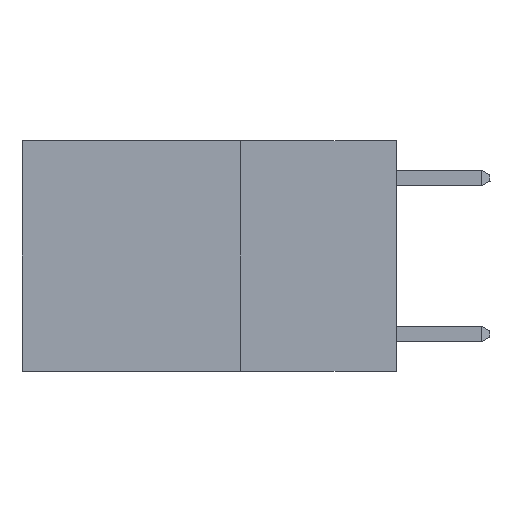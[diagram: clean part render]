
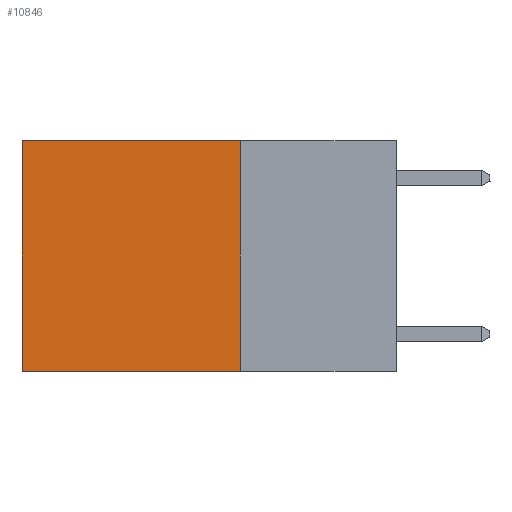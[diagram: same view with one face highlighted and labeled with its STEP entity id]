
A CAD part, left-side view. The second image highlights one B-rep face of the part: STEP entity #10846.
In plain terms, the highlighted planar face has unit normal (-1, 0, 0).
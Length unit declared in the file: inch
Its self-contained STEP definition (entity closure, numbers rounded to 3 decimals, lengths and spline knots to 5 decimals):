
#853 = EDGE_CURVE ( 'NONE', #4057, #1372, #12557, .T. ) ;
#1372 = VERTEX_POINT ( 'NONE', #14731 ) ;
#1392 = FACE_OUTER_BOUND ( 'NONE', #7752, .T. ) ;
#2398 = EDGE_CURVE ( 'NONE', #14390, #4057, #13760, .T. ) ;
#2443 = ORIENTED_EDGE ( 'NONE', *, *, #853, .F. ) ;
#2927 = CARTESIAN_POINT ( 'NONE',  ( 0.2625, 0.25, -0.37 ) ) ;
#2970 = LINE ( 'NONE', #14959, #9417 ) ;
#3280 = ORIENTED_EDGE ( 'NONE', *, *, #3383, .T. ) ;
#3383 = EDGE_CURVE ( 'NONE', #14390, #9085, #14247, .T. ) ;
#3995 = DIRECTION ( 'NONE',  ( 0., 0., -1. ) ) ;
#4057 = VERTEX_POINT ( 'NONE', #10858 ) ;
#6278 = VECTOR ( 'NONE', #7121, 39.37008 ) ;
#6749 = EDGE_CURVE ( 'NONE', #9085, #1372, #2970, .T. ) ;
#7121 = DIRECTION ( 'NONE',  ( 0., 1., 0. ) ) ;
#7445 = CARTESIAN_POINT ( 'NONE',  ( 0.2625, 0.25, 0. ) ) ;
#7752 = EDGE_LOOP ( 'NONE', ( #8179, #2443, #12807, #3280 ) ) ;
#8096 = CARTESIAN_POINT ( 'NONE',  ( 0.2625, 0.25, 0. ) ) ;
#8179 = ORIENTED_EDGE ( 'NONE', *, *, #6749, .T. ) ;
#8688 = DIRECTION ( 'NONE',  ( 0., 0., -1. ) ) ;
#9085 = VERTEX_POINT ( 'NONE', #13695 ) ;
#9323 = DIRECTION ( 'NONE',  ( 0., 0., -1. ) ) ;
#9417 = VECTOR ( 'NONE', #9323, 39.37008 ) ;
#10846 = ADVANCED_FACE ( 'NONE', ( #1392 ), #13202, .F. ) ;
#10858 = CARTESIAN_POINT ( 'NONE',  ( 0.2625, 0.25, -0.37 ) ) ;
#11094 = VECTOR ( 'NONE', #3995, 39.37008 ) ;
#11392 = CARTESIAN_POINT ( 'NONE',  ( 0.2625, 0.25, 0. ) ) ;
#11477 = AXIS2_PLACEMENT_3D ( 'NONE', #7445, #15449, #8688 ) ;
#11571 = DIRECTION ( 'NONE',  ( 0., 1., 0. ) ) ;
#12557 = LINE ( 'NONE', #2927, #6278 ) ;
#12807 = ORIENTED_EDGE ( 'NONE', *, *, #2398, .F. ) ;
#13202 = PLANE ( 'NONE',  #11477 ) ;
#13223 = CARTESIAN_POINT ( 'NONE',  ( 0.2625, 0.25, 0. ) ) ;
#13695 = CARTESIAN_POINT ( 'NONE',  ( 0.2625, 0.6, 0. ) ) ;
#13760 = LINE ( 'NONE', #11392, #11094 ) ;
#13883 = VECTOR ( 'NONE', #11571, 39.37008 ) ;
#14247 = LINE ( 'NONE', #8096, #13883 ) ;
#14390 = VERTEX_POINT ( 'NONE', #13223 ) ;
#14731 = CARTESIAN_POINT ( 'NONE',  ( 0.2625, 0.6, -0.37 ) ) ;
#14959 = CARTESIAN_POINT ( 'NONE',  ( 0.2625, 0.6, 0. ) ) ;
#15449 = DIRECTION ( 'NONE',  ( 1., 0., 0. ) ) ;
